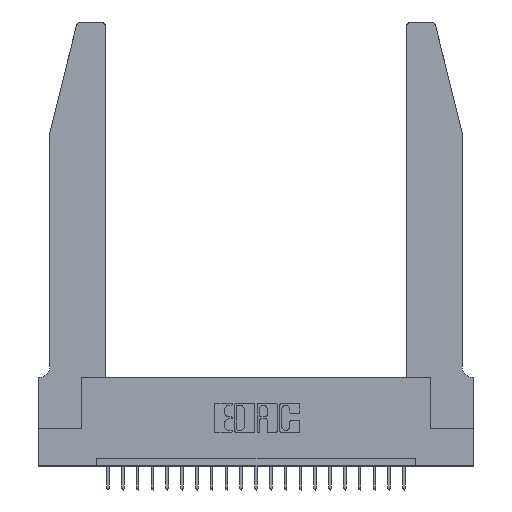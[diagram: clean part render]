
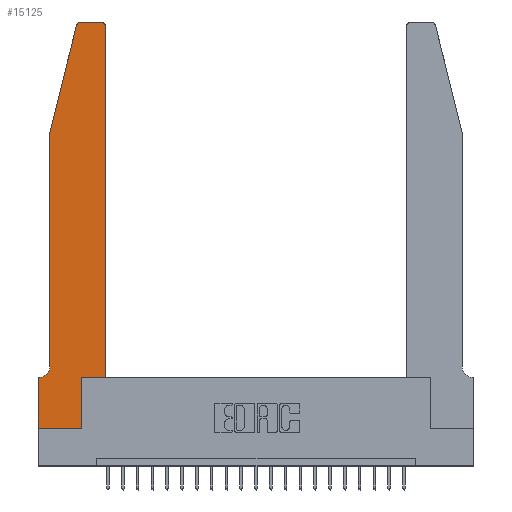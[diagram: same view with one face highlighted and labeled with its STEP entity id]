
A CAD part, top view. The second image highlights one B-rep face of the part: STEP entity #15125.
In plain terms, the highlighted planar face has unit normal (0, 0, 1).
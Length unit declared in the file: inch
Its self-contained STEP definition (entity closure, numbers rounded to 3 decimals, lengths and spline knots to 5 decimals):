
#103 = VECTOR ( 'NONE', #10000, 39.37008 ) ;
#175 = LINE ( 'NONE', #2005, #16355 ) ;
#393 = ORIENTED_EDGE ( 'NONE', *, *, #20900, .T. ) ;
#670 = CARTESIAN_POINT ( 'NONE',  ( 0.25487, 2.72718, 0.37 ) ) ;
#764 = CIRCLE ( 'NONE', #848, 0.03 ) ;
#848 = AXIS2_PLACEMENT_3D ( 'NONE', #7729, #14887, #13304 ) ;
#946 = CARTESIAN_POINT ( 'NONE',  ( 0., 0., 0.37 ) ) ;
#963 = LINE ( 'NONE', #22569, #103 ) ;
#1061 = ORIENTED_EDGE ( 'NONE', *, *, #22068, .T. ) ;
#1159 = CARTESIAN_POINT ( 'NONE',  ( 0.4505, 0.35, 0.37 ) ) ;
#1495 = DIRECTION ( 'NONE',  ( -1., 0., 0. ) ) ;
#1528 = CARTESIAN_POINT ( 'NONE',  ( 0.0755, 0.35, 0.37 ) ) ;
#1570 = VERTEX_POINT ( 'NONE', #21288 ) ;
#1829 = VERTEX_POINT ( 'NONE', #5585 ) ;
#2005 = CARTESIAN_POINT ( 'NONE',  ( 0.0755, 2., 0.37 ) ) ;
#2029 = CARTESIAN_POINT ( 'NONE',  ( 0.0755, 0.42, 0.37 ) ) ;
#3078 = DIRECTION ( 'NONE',  ( -1., 0., 0. ) ) ;
#3259 = VECTOR ( 'NONE', #16526, 39.37008 ) ;
#3471 = VECTOR ( 'NONE', #15044, 39.37008 ) ;
#3773 = EDGE_CURVE ( 'NONE', #20247, #6953, #16392, .T. ) ;
#3963 = ORIENTED_EDGE ( 'NONE', *, *, #9852, .T. ) ;
#4066 = ORIENTED_EDGE ( 'NONE', *, *, #18088, .T. ) ;
#4072 = EDGE_CURVE ( 'NONE', #1829, #11641, #10331, .T. ) ;
#4110 = DIRECTION ( 'NONE',  ( 0., 0., 1. ) ) ;
#4402 = LINE ( 'NONE', #21946, #3259 ) ;
#4899 = ORIENTED_EDGE ( 'NONE', *, *, #5217, .T. ) ;
#4948 = VERTEX_POINT ( 'NONE', #20269 ) ;
#5164 = CARTESIAN_POINT ( 'NONE',  ( 0.0055, 0.35, 0.37 ) ) ;
#5217 = EDGE_CURVE ( 'NONE', #6953, #4948, #5475, .T. ) ;
#5475 = LINE ( 'NONE', #1528, #6870 ) ;
#5585 = CARTESIAN_POINT ( 'NONE',  ( 0.4505, 0.35, 0.37 ) ) ;
#5596 = VERTEX_POINT ( 'NONE', #670 ) ;
#5859 = EDGE_CURVE ( 'NONE', #21420, #21945, #20542, .T. ) ;
#6102 = DIRECTION ( 'NONE',  ( 0., 1., 0. ) ) ;
#6301 = CARTESIAN_POINT ( 'NONE',  ( 0.0055, 0.42, 0.37 ) ) ;
#6339 = LINE ( 'NONE', #18937, #15219 ) ;
#6400 = CARTESIAN_POINT ( 'NONE',  ( 0.4505, 2.72, 0.37 ) ) ;
#6580 = DIRECTION ( 'NONE',  ( 1., 0., 0. ) ) ;
#6794 = ORIENTED_EDGE ( 'NONE', *, *, #5859, .T. ) ;
#6870 = VECTOR ( 'NONE', #8838, 39.37008 ) ;
#6953 = VERTEX_POINT ( 'NONE', #5164 ) ;
#7437 = AXIS2_PLACEMENT_3D ( 'NONE', #14039, #10587, #6580 ) ;
#7729 = CARTESIAN_POINT ( 'NONE',  ( 0.284, 2.72, 0.37 ) ) ;
#7809 = CARTESIAN_POINT ( 'NONE',  ( 0.4505, 0.35, 0.37 ) ) ;
#8838 = DIRECTION ( 'NONE',  ( -1., 0., 0. ) ) ;
#9025 = FACE_OUTER_BOUND ( 'NONE', #11949, .T. ) ;
#9315 = ORIENTED_EDGE ( 'NONE', *, *, #12613, .T. ) ;
#9629 = DIRECTION ( 'NONE',  ( 1., 0., 0. ) ) ;
#9852 = EDGE_CURVE ( 'NONE', #4948, #1570, #4402, .T. ) ;
#10000 = DIRECTION ( 'NONE',  ( -0.239, -0.971, 0. ) ) ;
#10331 = LINE ( 'NONE', #1159, #21693 ) ;
#10587 = DIRECTION ( 'NONE',  ( 0., 0., 1. ) ) ;
#11038 = DIRECTION ( 'NONE',  ( 0., -1., 0. ) ) ;
#11551 = CARTESIAN_POINT ( 'NONE',  ( 0.284, 2.75, 0.37 ) ) ;
#11641 = VERTEX_POINT ( 'NONE', #6400 ) ;
#11949 = EDGE_LOOP ( 'NONE', ( #6794, #19222, #1061, #393, #21163, #4899, #3963, #9315, #4066, #14069, #20951, #13868 ) ) ;
#12375 = DIRECTION ( 'NONE',  ( 0., 0., -1. ) ) ;
#12613 = EDGE_CURVE ( 'NONE', #1570, #18776, #19407, .T. ) ;
#13166 = CARTESIAN_POINT ( 'NONE',  ( 0.4205, 2.72, 0.37 ) ) ;
#13173 = EDGE_CURVE ( 'NONE', #14879, #1829, #17695, .T. ) ;
#13304 = DIRECTION ( 'NONE',  ( 1., 0., 0. ) ) ;
#13868 = ORIENTED_EDGE ( 'NONE', *, *, #14192, .T. ) ;
#13869 = AXIS2_PLACEMENT_3D ( 'NONE', #13166, #4110, #9629 ) ;
#13889 = CARTESIAN_POINT ( 'NONE',  ( 0.2865, 0., 0.37 ) ) ;
#14022 = VECTOR ( 'NONE', #21086, 39.37008 ) ;
#14039 = CARTESIAN_POINT ( 'NONE',  ( 0., 0.35, 0.37 ) ) ;
#14069 = ORIENTED_EDGE ( 'NONE', *, *, #13173, .T. ) ;
#14192 = EDGE_CURVE ( 'NONE', #11641, #21420, #19924, .T. ) ;
#14569 = VECTOR ( 'NONE', #3078, 39.37008 ) ;
#14879 = VERTEX_POINT ( 'NONE', #18577 ) ;
#14887 = DIRECTION ( 'NONE',  ( 0., 0., 1. ) ) ;
#15044 = DIRECTION ( 'NONE',  ( 1., 0., 0. ) ) ;
#15125 = ADVANCED_FACE ( 'NONE', ( #9025 ), #16023, .T. ) ;
#15219 = VECTOR ( 'NONE', #6102, 39.37008 ) ;
#15776 = DIRECTION ( 'NONE',  ( 0., 1., 0. ) ) ;
#16023 = PLANE ( 'NONE',  #7437 ) ;
#16355 = VECTOR ( 'NONE', #11038, 39.37008 ) ;
#16392 = CIRCLE ( 'NONE', #19077, 0.07 ) ;
#16526 = DIRECTION ( 'NONE',  ( 0., -1., 0. ) ) ;
#17169 = EDGE_CURVE ( 'NONE', #21945, #5596, #764, .T. ) ;
#17695 = LINE ( 'NONE', #7809, #3471 ) ;
#17697 = VERTEX_POINT ( 'NONE', #19487 ) ;
#18088 = EDGE_CURVE ( 'NONE', #18776, #14879, #6339, .T. ) ;
#18577 = CARTESIAN_POINT ( 'NONE',  ( 0.2865, 0.35, 0.37 ) ) ;
#18776 = VERTEX_POINT ( 'NONE', #13889 ) ;
#18937 = CARTESIAN_POINT ( 'NONE',  ( 0.2865, 0.35, 0.37 ) ) ;
#19077 = AXIS2_PLACEMENT_3D ( 'NONE', #6301, #12375, #1495 ) ;
#19222 = ORIENTED_EDGE ( 'NONE', *, *, #17169, .T. ) ;
#19407 = LINE ( 'NONE', #946, #14022 ) ;
#19487 = CARTESIAN_POINT ( 'NONE',  ( 0.0755, 2., 0.37 ) ) ;
#19924 = CIRCLE ( 'NONE', #13869, 0.03 ) ;
#20247 = VERTEX_POINT ( 'NONE', #2029 ) ;
#20269 = CARTESIAN_POINT ( 'NONE',  ( 0., 0.35, 0.37 ) ) ;
#20542 = LINE ( 'NONE', #21092, #14569 ) ;
#20900 = EDGE_CURVE ( 'NONE', #17697, #20247, #175, .T. ) ;
#20951 = ORIENTED_EDGE ( 'NONE', *, *, #4072, .T. ) ;
#21086 = DIRECTION ( 'NONE',  ( 1., 0., 0. ) ) ;
#21092 = CARTESIAN_POINT ( 'NONE',  ( 0.2605, 2.75, 0.37 ) ) ;
#21163 = ORIENTED_EDGE ( 'NONE', *, *, #3773, .T. ) ;
#21288 = CARTESIAN_POINT ( 'NONE',  ( 0., 0., 0.37 ) ) ;
#21420 = VERTEX_POINT ( 'NONE', #22514 ) ;
#21693 = VECTOR ( 'NONE', #15776, 39.37008 ) ;
#21945 = VERTEX_POINT ( 'NONE', #11551 ) ;
#21946 = CARTESIAN_POINT ( 'NONE',  ( 0., 0., 0.37 ) ) ;
#22068 = EDGE_CURVE ( 'NONE', #5596, #17697, #963, .T. ) ;
#22514 = CARTESIAN_POINT ( 'NONE',  ( 0.4205, 2.75, 0.37 ) ) ;
#22569 = CARTESIAN_POINT ( 'NONE',  ( 0.0755, 2., 0.37 ) ) ;
